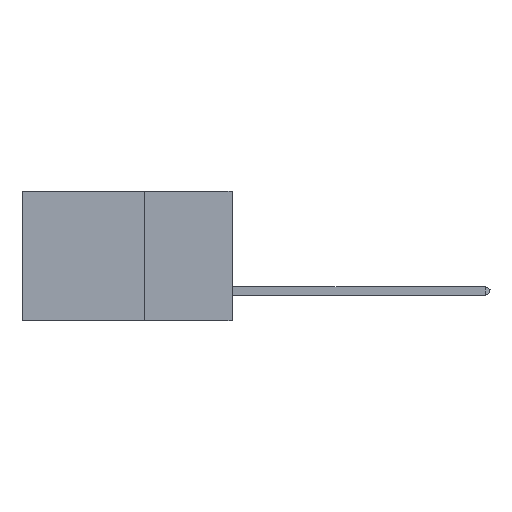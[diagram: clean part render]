
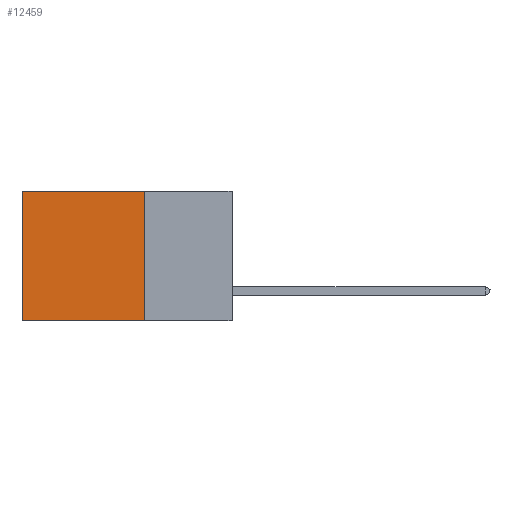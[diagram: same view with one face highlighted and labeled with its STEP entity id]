
A CAD part, left-side view. The second image highlights one B-rep face of the part: STEP entity #12459.
In plain terms, the highlighted planar face has unit normal (-1, 0, 0).
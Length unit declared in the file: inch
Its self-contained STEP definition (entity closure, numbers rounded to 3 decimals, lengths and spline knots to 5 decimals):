
#1534 = ORIENTED_EDGE ( 'NONE', *, *, #25192, .F. ) ;
#1557 = CARTESIAN_POINT ( 'NONE',  ( 0.2875, 0.25, 0. ) ) ;
#1704 = DIRECTION ( 'NONE',  ( 0., 0., -1. ) ) ;
#2649 = ORIENTED_EDGE ( 'NONE', *, *, #3263, .T. ) ;
#3144 = CARTESIAN_POINT ( 'NONE',  ( 0.2875, 0.25, -0.37 ) ) ;
#3263 = EDGE_CURVE ( 'NONE', #22717, #29661, #7099, .T. ) ;
#4250 = CARTESIAN_POINT ( 'NONE',  ( 0.2875, 0.6, 0. ) ) ;
#4557 = FACE_OUTER_BOUND ( 'NONE', #11044, .T. ) ;
#6551 = CARTESIAN_POINT ( 'NONE',  ( 0.2875, 0.25, 0. ) ) ;
#7099 = LINE ( 'NONE', #6551, #28557 ) ;
#8241 = EDGE_CURVE ( 'NONE', #22717, #19094, #23727, .T. ) ;
#8337 = CARTESIAN_POINT ( 'NONE',  ( 0.2875, 0.25, 0. ) ) ;
#11044 = EDGE_LOOP ( 'NONE', ( #15546, #1534, #36877, #2649 ) ) ;
#12459 = ADVANCED_FACE ( 'NONE', ( #4557 ), #22031, .F. ) ;
#14561 = VERTEX_POINT ( 'NONE', #18989 ) ;
#15546 = ORIENTED_EDGE ( 'NONE', *, *, #40124, .T. ) ;
#17384 = DIRECTION ( 'NONE',  ( 0., 0., -1. ) ) ;
#18989 = CARTESIAN_POINT ( 'NONE',  ( 0.2875, 0.6, -0.37 ) ) ;
#19094 = VERTEX_POINT ( 'NONE', #20646 ) ;
#20646 = CARTESIAN_POINT ( 'NONE',  ( 0.2875, 0.25, -0.37 ) ) ;
#21421 = DIRECTION ( 'NONE',  ( 1., 0., 0. ) ) ;
#22031 = PLANE ( 'NONE',  #35054 ) ;
#22717 = VERTEX_POINT ( 'NONE', #37918 ) ;
#23727 = LINE ( 'NONE', #1557, #39892 ) ;
#25192 = EDGE_CURVE ( 'NONE', #19094, #14561, #34068, .T. ) ;
#25248 = VECTOR ( 'NONE', #29574, 39.37008 ) ;
#28184 = DIRECTION ( 'NONE',  ( 0., 0., -1. ) ) ;
#28557 = VECTOR ( 'NONE', #29907, 39.37008 ) ;
#29574 = DIRECTION ( 'NONE',  ( 0., 1., 0. ) ) ;
#29661 = VERTEX_POINT ( 'NONE', #35106 ) ;
#29907 = DIRECTION ( 'NONE',  ( 0., 1., 0. ) ) ;
#30363 = LINE ( 'NONE', #4250, #37105 ) ;
#34068 = LINE ( 'NONE', #3144, #25248 ) ;
#35054 = AXIS2_PLACEMENT_3D ( 'NONE', #8337, #21421, #1704 ) ;
#35106 = CARTESIAN_POINT ( 'NONE',  ( 0.2875, 0.6, 0. ) ) ;
#36877 = ORIENTED_EDGE ( 'NONE', *, *, #8241, .F. ) ;
#37105 = VECTOR ( 'NONE', #17384, 39.37008 ) ;
#37918 = CARTESIAN_POINT ( 'NONE',  ( 0.2875, 0.25, 0. ) ) ;
#39892 = VECTOR ( 'NONE', #28184, 39.37008 ) ;
#40124 = EDGE_CURVE ( 'NONE', #29661, #14561, #30363, .T. ) ;
